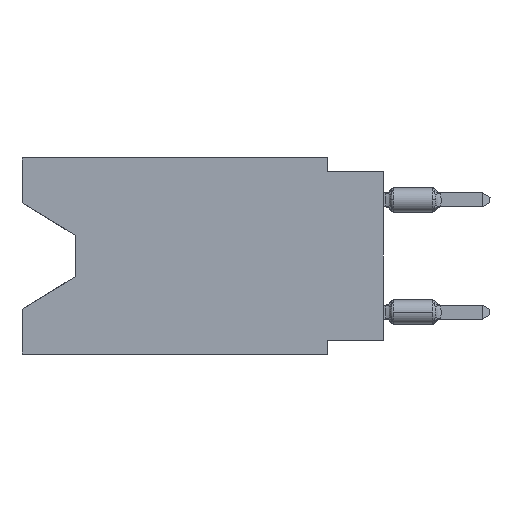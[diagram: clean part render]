
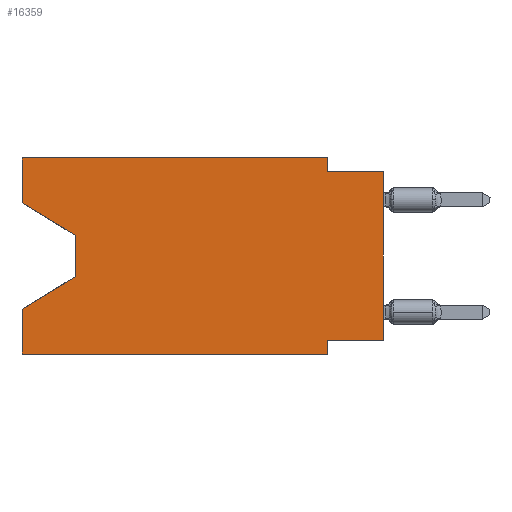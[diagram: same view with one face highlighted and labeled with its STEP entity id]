
A CAD part, left-side view. The second image highlights one B-rep face of the part: STEP entity #16359.
In plain terms, the highlighted planar face has unit normal (-1, 0, 0).
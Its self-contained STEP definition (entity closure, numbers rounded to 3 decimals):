
#145 = LINE ( 'NONE', #2242, #13220 ) ;
#655 = LINE ( 'NONE', #8985, #10112 ) ;
#731 = CARTESIAN_POINT ( 'NONE',  ( 0., 0., -8.255 ) ) ;
#804 = FACE_OUTER_BOUND ( 'NONE', #7119, .T. ) ;
#849 = CARTESIAN_POINT ( 'NONE',  ( 0., 0., -0.635 ) ) ;
#961 = CARTESIAN_POINT ( 'NONE',  ( 0., 16.383, -8.89 ) ) ;
#1482 = ORIENTED_EDGE ( 'NONE', *, *, #2605, .F. ) ;
#1485 = EDGE_CURVE ( 'NONE', #9134, #25553, #655, .T. ) ;
#1797 = LINE ( 'NONE', #18717, #2090 ) ;
#2090 = VECTOR ( 'NONE', #16643, 1000. ) ;
#2242 = CARTESIAN_POINT ( 'NONE',  ( 0., 13.97, -5.385 ) ) ;
#2574 = CARTESIAN_POINT ( 'NONE',  ( 0., 2.54, 0. ) ) ;
#2605 = EDGE_CURVE ( 'NONE', #22830, #22102, #24598, .T. ) ;
#2662 = CARTESIAN_POINT ( 'NONE',  ( 0., 2.54, -8.89 ) ) ;
#2757 = LINE ( 'NONE', #4841, #14852 ) ;
#3874 = CARTESIAN_POINT ( 'NONE',  ( 0., 16.383, -8.89 ) ) ;
#4715 = EDGE_CURVE ( 'NONE', #26576, #18484, #13037, .T. ) ;
#4841 = CARTESIAN_POINT ( 'NONE',  ( 0., 13.97, -3.505 ) ) ;
#5958 = EDGE_CURVE ( 'NONE', #9134, #22102, #15412, .T. ) ;
#6100 = LINE ( 'NONE', #9738, #11456 ) ;
#6843 = VERTEX_POINT ( 'NONE', #731 ) ;
#7119 = EDGE_LOOP ( 'NONE', ( #23888, #21483, #27034, #15207, #17641, #1482, #24543, #22659, #19618, #18128, #16981, #17178 ) ) ;
#7477 = PLANE ( 'NONE',  #8273 ) ;
#7630 = EDGE_CURVE ( 'NONE', #18484, #9971, #2757, .T. ) ;
#8078 = CARTESIAN_POINT ( 'NONE',  ( 0., 2.54, -8.89 ) ) ;
#8273 = AXIS2_PLACEMENT_3D ( 'NONE', #19671, #13735, #13445 ) ;
#8321 = DIRECTION ( 'NONE',  ( 0., -0.855, -0.519 ) ) ;
#8916 = CARTESIAN_POINT ( 'NONE',  ( 0., 0., -0.635 ) ) ;
#8985 = CARTESIAN_POINT ( 'NONE',  ( 0., 16.383, 0. ) ) ;
#9134 = VERTEX_POINT ( 'NONE', #3874 ) ;
#9589 = CARTESIAN_POINT ( 'NONE',  ( 0., 0., 0. ) ) ;
#9738 = CARTESIAN_POINT ( 'NONE',  ( 0., 0., -8.255 ) ) ;
#9971 = VERTEX_POINT ( 'NONE', #25294 ) ;
#10112 = VECTOR ( 'NONE', #23686, 1000. ) ;
#10370 = CARTESIAN_POINT ( 'NONE',  ( 0., 16.383, -2.038 ) ) ;
#10703 = DIRECTION ( 'NONE',  ( 0., 0.855, -0.519 ) ) ;
#11431 = EDGE_CURVE ( 'NONE', #6843, #22830, #6100, .T. ) ;
#11456 = VECTOR ( 'NONE', #26656, 1000. ) ;
#11485 = VECTOR ( 'NONE', #8321, 1000. ) ;
#12137 = DIRECTION ( 'NONE',  ( 0., -1., 0. ) ) ;
#12444 = LINE ( 'NONE', #21293, #26603 ) ;
#12828 = EDGE_CURVE ( 'NONE', #13127, #21015, #23737, .T. ) ;
#13037 = LINE ( 'NONE', #27339, #11485 ) ;
#13127 = VERTEX_POINT ( 'NONE', #13140 ) ;
#13140 = CARTESIAN_POINT ( 'NONE',  ( 0., 2.54, -0.635 ) ) ;
#13220 = VECTOR ( 'NONE', #10703, 1000. ) ;
#13445 = DIRECTION ( 'NONE',  ( 0., 0., -1. ) ) ;
#13572 = EDGE_CURVE ( 'NONE', #23866, #13127, #12444, .T. ) ;
#13735 = DIRECTION ( 'NONE',  ( 1., 0., 0. ) ) ;
#13866 = EDGE_CURVE ( 'NONE', #26674, #23866, #22542, .T. ) ;
#14240 = VECTOR ( 'NONE', #14690, 1000. ) ;
#14690 = DIRECTION ( 'NONE',  ( 0., 0., 1. ) ) ;
#14810 = LINE ( 'NONE', #9589, #14240 ) ;
#14852 = VECTOR ( 'NONE', #23695, 1000. ) ;
#15207 = ORIENTED_EDGE ( 'NONE', *, *, #1485, .F. ) ;
#15412 = LINE ( 'NONE', #961, #21922 ) ;
#16322 = CARTESIAN_POINT ( 'NONE',  ( 0., 2.54, -8.255 ) ) ;
#16359 = ADVANCED_FACE ( 'NONE', ( #804 ), #7477, .F. ) ;
#16643 = DIRECTION ( 'NONE',  ( 0., 0., 1. ) ) ;
#16981 = ORIENTED_EDGE ( 'NONE', *, *, #13866, .F. ) ;
#17178 = ORIENTED_EDGE ( 'NONE', *, *, #20084, .F. ) ;
#17341 = CARTESIAN_POINT ( 'NONE',  ( 0., 13.97, -3.505 ) ) ;
#17641 = ORIENTED_EDGE ( 'NONE', *, *, #5958, .T. ) ;
#17895 = DIRECTION ( 'NONE',  ( 0., -1., 0. ) ) ;
#18128 = ORIENTED_EDGE ( 'NONE', *, *, #13572, .F. ) ;
#18201 = VECTOR ( 'NONE', #12137, 1000. ) ;
#18372 = CARTESIAN_POINT ( 'NONE',  ( 0., 16.383, 0. ) ) ;
#18484 = VERTEX_POINT ( 'NONE', #17341 ) ;
#18639 = DIRECTION ( 'NONE',  ( 0., 0., -1. ) ) ;
#18717 = CARTESIAN_POINT ( 'NONE',  ( 0., 16.383, 0. ) ) ;
#18943 = DIRECTION ( 'NONE',  ( 0., 0., -1. ) ) ;
#19618 = ORIENTED_EDGE ( 'NONE', *, *, #12828, .F. ) ;
#19671 = CARTESIAN_POINT ( 'NONE',  ( 0., 16.383, 0. ) ) ;
#20084 = EDGE_CURVE ( 'NONE', #26576, #26674, #1797, .T. ) ;
#21015 = VERTEX_POINT ( 'NONE', #8916 ) ;
#21293 = CARTESIAN_POINT ( 'NONE',  ( 0., 2.54, 0. ) ) ;
#21483 = ORIENTED_EDGE ( 'NONE', *, *, #7630, .T. ) ;
#21735 = CARTESIAN_POINT ( 'NONE',  ( 0., 16.383, 0. ) ) ;
#21922 = VECTOR ( 'NONE', #17895, 1000. ) ;
#22102 = VERTEX_POINT ( 'NONE', #2662 ) ;
#22116 = CARTESIAN_POINT ( 'NONE',  ( 0., 16.383, -6.852 ) ) ;
#22542 = LINE ( 'NONE', #18372, #18201 ) ;
#22659 = ORIENTED_EDGE ( 'NONE', *, *, #26566, .T. ) ;
#22830 = VERTEX_POINT ( 'NONE', #16322 ) ;
#22987 = VECTOR ( 'NONE', #18639, 1000. ) ;
#23686 = DIRECTION ( 'NONE',  ( 0., 0., 1. ) ) ;
#23695 = DIRECTION ( 'NONE',  ( 0., 0., -1. ) ) ;
#23737 = LINE ( 'NONE', #849, #26583 ) ;
#23866 = VERTEX_POINT ( 'NONE', #2574 ) ;
#23888 = ORIENTED_EDGE ( 'NONE', *, *, #4715, .T. ) ;
#24543 = ORIENTED_EDGE ( 'NONE', *, *, #11431, .F. ) ;
#24598 = LINE ( 'NONE', #8078, #22987 ) ;
#24655 = EDGE_CURVE ( 'NONE', #9971, #25553, #145, .T. ) ;
#25294 = CARTESIAN_POINT ( 'NONE',  ( 0., 13.97, -5.385 ) ) ;
#25553 = VERTEX_POINT ( 'NONE', #22116 ) ;
#25691 = DIRECTION ( 'NONE',  ( 0., -1., 0. ) ) ;
#26566 = EDGE_CURVE ( 'NONE', #6843, #21015, #14810, .T. ) ;
#26576 = VERTEX_POINT ( 'NONE', #10370 ) ;
#26583 = VECTOR ( 'NONE', #25691, 1000. ) ;
#26603 = VECTOR ( 'NONE', #18943, 1000. ) ;
#26656 = DIRECTION ( 'NONE',  ( 0., 1., 0. ) ) ;
#26674 = VERTEX_POINT ( 'NONE', #21735 ) ;
#27034 = ORIENTED_EDGE ( 'NONE', *, *, #24655, .T. ) ;
#27339 = CARTESIAN_POINT ( 'NONE',  ( 0., 16.383, -2.038 ) ) ;
